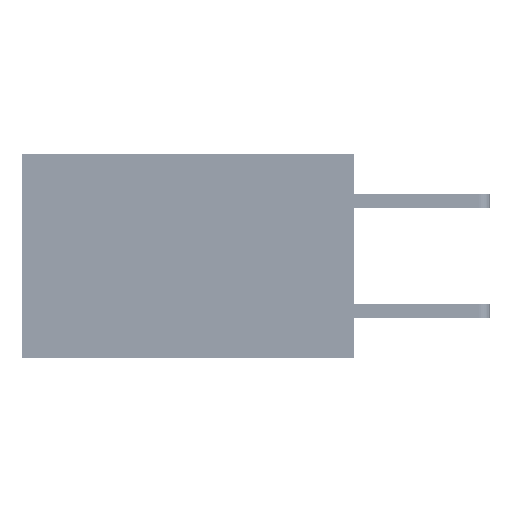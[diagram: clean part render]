
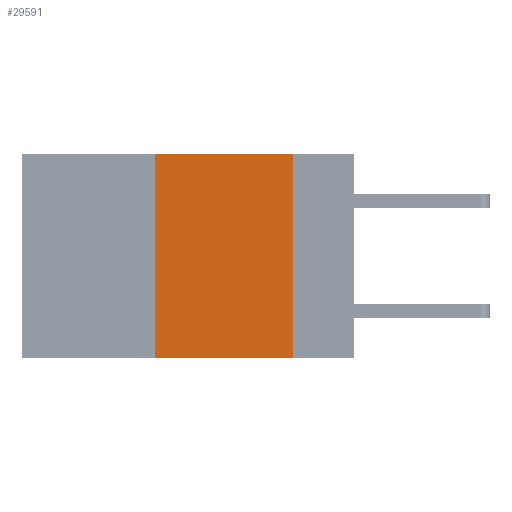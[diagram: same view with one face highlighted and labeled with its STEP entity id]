
A CAD part, left-side view. The second image highlights one B-rep face of the part: STEP entity #29591.
In plain terms, the highlighted planar face has unit normal (-1, 0, 0).
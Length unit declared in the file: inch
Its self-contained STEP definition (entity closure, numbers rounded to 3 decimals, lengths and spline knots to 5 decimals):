
#839 = CARTESIAN_POINT ( 'NONE',  ( 0., 0.11, 0. ) ) ;
#911 = DIRECTION ( 'NONE',  ( 1., 0., 0. ) ) ;
#3202 = CARTESIAN_POINT ( 'NONE',  ( 0., 0.36, 0. ) ) ;
#3845 = ORIENTED_EDGE ( 'NONE', *, *, #50619, .F. ) ;
#5112 = DIRECTION ( 'NONE',  ( 0., 0., -1. ) ) ;
#5150 = EDGE_CURVE ( 'NONE', #25271, #17442, #33810, .T. ) ;
#5523 = CARTESIAN_POINT ( 'NONE',  ( 0., 0.36, 0. ) ) ;
#5712 = LINE ( 'NONE', #34782, #36626 ) ;
#6486 = VECTOR ( 'NONE', #16644, 39.37008 ) ;
#6501 = VERTEX_POINT ( 'NONE', #9938 ) ;
#7421 = EDGE_CURVE ( 'NONE', #25271, #8850, #5712, .T. ) ;
#8077 = ORIENTED_EDGE ( 'NONE', *, *, #5150, .F. ) ;
#8850 = VERTEX_POINT ( 'NONE', #34318 ) ;
#9580 = VECTOR ( 'NONE', #40978, 39.37008 ) ;
#9938 = CARTESIAN_POINT ( 'NONE',  ( 0., 0.11, 0. ) ) ;
#12685 = CARTESIAN_POINT ( 'NONE',  ( 0., 0.6, 0. ) ) ;
#15061 = DIRECTION ( 'NONE',  ( 0., -1., 0. ) ) ;
#16644 = DIRECTION ( 'NONE',  ( 0., -1., 0. ) ) ;
#17442 = VERTEX_POINT ( 'NONE', #3202 ) ;
#20187 = CARTESIAN_POINT ( 'NONE',  ( 0., 0.36, -0.37 ) ) ;
#20878 = EDGE_CURVE ( 'NONE', #6501, #8850, #47983, .T. ) ;
#21443 = ORIENTED_EDGE ( 'NONE', *, *, #7421, .T. ) ;
#24797 = PLANE ( 'NONE',  #48735 ) ;
#25271 = VERTEX_POINT ( 'NONE', #20187 ) ;
#28824 = LINE ( 'NONE', #12685, #6486 ) ;
#28935 = CARTESIAN_POINT ( 'NONE',  ( 0., 0.6, 0. ) ) ;
#29591 = ADVANCED_FACE ( 'NONE', ( #37777 ), #24797, .F. ) ;
#33810 = LINE ( 'NONE', #5523, #9580 ) ;
#34010 = EDGE_LOOP ( 'NONE', ( #37091, #3845, #8077, #21443 ) ) ;
#34318 = CARTESIAN_POINT ( 'NONE',  ( 0., 0.11, -0.37 ) ) ;
#34782 = CARTESIAN_POINT ( 'NONE',  ( 0., 0.6, -0.37 ) ) ;
#36626 = VECTOR ( 'NONE', #15061, 39.37008 ) ;
#37091 = ORIENTED_EDGE ( 'NONE', *, *, #20878, .F. ) ;
#37777 = FACE_OUTER_BOUND ( 'NONE', #34010, .T. ) ;
#40978 = DIRECTION ( 'NONE',  ( 0., 0., 1. ) ) ;
#43656 = VECTOR ( 'NONE', #5112, 39.37008 ) ;
#47983 = LINE ( 'NONE', #839, #43656 ) ;
#48292 = DIRECTION ( 'NONE',  ( 0., 0., -1. ) ) ;
#48735 = AXIS2_PLACEMENT_3D ( 'NONE', #28935, #911, #48292 ) ;
#50619 = EDGE_CURVE ( 'NONE', #17442, #6501, #28824, .T. ) ;
